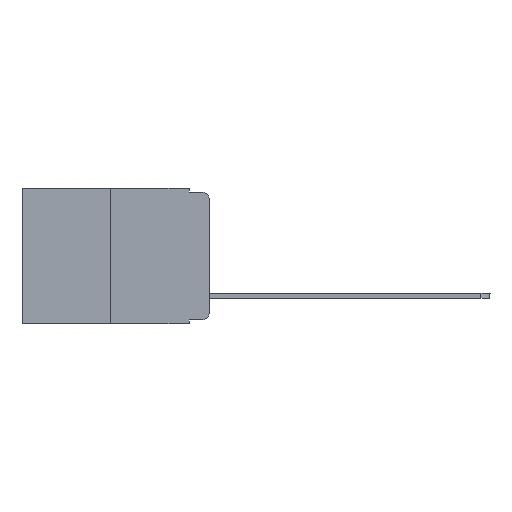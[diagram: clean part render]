
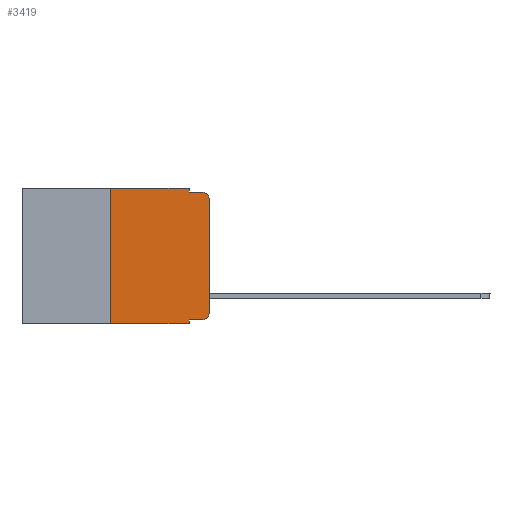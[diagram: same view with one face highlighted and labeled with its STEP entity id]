
A CAD part, left-side view. The second image highlights one B-rep face of the part: STEP entity #3419.
In plain terms, the highlighted planar face has unit normal (-1, 0, 0).
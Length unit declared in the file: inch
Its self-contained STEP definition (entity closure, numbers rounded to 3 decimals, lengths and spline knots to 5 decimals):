
#386 = DIRECTION ( 'NONE',  ( 0., -1., 0. ) ) ;
#850 = ORIENTED_EDGE ( 'NONE', *, *, #2963, .F. ) ;
#1186 = CARTESIAN_POINT ( 'NONE',  ( 0., 0.02, -0.333 ) ) ;
#1317 = VERTEX_POINT ( 'NONE', #8424 ) ;
#1328 = CARTESIAN_POINT ( 'NONE',  ( 0., 0.02, -0.313 ) ) ;
#1638 = AXIS2_PLACEMENT_3D ( 'NONE', #11266, #3625, #21027 ) ;
#1737 = DIRECTION ( 'NONE',  ( 0., 0., -1. ) ) ;
#1816 = PLANE ( 'NONE',  #14323 ) ;
#2111 = CARTESIAN_POINT ( 'NONE',  ( 0., 0.473, 0. ) ) ;
#2673 = VECTOR ( 'NONE', #6507, 39.37008 ) ;
#2772 = EDGE_CURVE ( 'NONE', #17605, #16877, #12616, .T. ) ;
#2912 = LINE ( 'NONE', #18520, #10116 ) ;
#2963 = EDGE_CURVE ( 'NONE', #8290, #1317, #24633, .T. ) ;
#3319 = CARTESIAN_POINT ( 'NONE',  ( 0., 0.25, -0.343 ) ) ;
#3368 = LINE ( 'NONE', #15647, #24435 ) ;
#3419 = ADVANCED_FACE ( 'NONE', ( #14100 ), #1816, .F. ) ;
#3489 = ORIENTED_EDGE ( 'NONE', *, *, #8523, .F. ) ;
#3625 = DIRECTION ( 'NONE',  ( -1., 0., 0. ) ) ;
#3786 = ORIENTED_EDGE ( 'NONE', *, *, #5495, .T. ) ;
#3880 = VERTEX_POINT ( 'NONE', #7819 ) ;
#4097 = VERTEX_POINT ( 'NONE', #4780 ) ;
#4254 = VECTOR ( 'NONE', #16210, 39.37008 ) ;
#4737 = CARTESIAN_POINT ( 'NONE',  ( 0., 0., -0.03 ) ) ;
#4780 = CARTESIAN_POINT ( 'NONE',  ( 0., 0.02, -0.01 ) ) ;
#4804 = ORIENTED_EDGE ( 'NONE', *, *, #19034, .T. ) ;
#5077 = EDGE_CURVE ( 'NONE', #17605, #7780, #19011, .T. ) ;
#5107 = DIRECTION ( 'NONE',  ( -1., 0., 0. ) ) ;
#5423 = CARTESIAN_POINT ( 'NONE',  ( 0., 0.473, 0. ) ) ;
#5495 = EDGE_CURVE ( 'NONE', #16734, #4097, #6612, .T. ) ;
#6049 = VERTEX_POINT ( 'NONE', #13752 ) ;
#6392 = ORIENTED_EDGE ( 'NONE', *, *, #20083, .F. ) ;
#6507 = DIRECTION ( 'NONE',  ( 0., -1., 0. ) ) ;
#6580 = AXIS2_PLACEMENT_3D ( 'NONE', #1328, #5107, #6944 ) ;
#6612 = CIRCLE ( 'NONE', #1638, 0.02 ) ;
#6631 = VECTOR ( 'NONE', #13876, 39.37008 ) ;
#6944 = DIRECTION ( 'NONE',  ( 0., 0., -1. ) ) ;
#7354 = DIRECTION ( 'NONE',  ( 1., 0., 0. ) ) ;
#7780 = VERTEX_POINT ( 'NONE', #8704 ) ;
#7819 = CARTESIAN_POINT ( 'NONE',  ( 0., 0., -0.313 ) ) ;
#8290 = VERTEX_POINT ( 'NONE', #13399 ) ;
#8424 = CARTESIAN_POINT ( 'NONE',  ( 0., 0.051, 0. ) ) ;
#8523 = EDGE_CURVE ( 'NONE', #9885, #8290, #14919, .T. ) ;
#8704 = CARTESIAN_POINT ( 'NONE',  ( 0., 0.051, -0.343 ) ) ;
#8719 = ORIENTED_EDGE ( 'NONE', *, *, #17128, .F. ) ;
#9520 = DIRECTION ( 'NONE',  ( 0., 0., -1. ) ) ;
#9591 = VECTOR ( 'NONE', #11482, 39.37008 ) ;
#9613 = VECTOR ( 'NONE', #15052, 39.37008 ) ;
#9885 = VERTEX_POINT ( 'NONE', #3319 ) ;
#10116 = VECTOR ( 'NONE', #9520, 39.37008 ) ;
#11083 = CARTESIAN_POINT ( 'NONE',  ( 0., 0.051, -0.333 ) ) ;
#11266 = CARTESIAN_POINT ( 'NONE',  ( 0., 0.02, -0.03 ) ) ;
#11288 = CIRCLE ( 'NONE', #6580, 0.02 ) ;
#11372 = LINE ( 'NONE', #16880, #9591 ) ;
#11482 = DIRECTION ( 'NONE',  ( 0., 0., 1. ) ) ;
#11768 = LINE ( 'NONE', #16019, #6631 ) ;
#12616 = LINE ( 'NONE', #13467, #9613 ) ;
#13399 = CARTESIAN_POINT ( 'NONE',  ( 0., 0.25, 0. ) ) ;
#13467 = CARTESIAN_POINT ( 'NONE',  ( 0., 0.051, -0.333 ) ) ;
#13752 = CARTESIAN_POINT ( 'NONE',  ( 0., 0.051, -0.01 ) ) ;
#13791 = CARTESIAN_POINT ( 'NONE',  ( 0., 0.051, 0. ) ) ;
#13815 = ORIENTED_EDGE ( 'NONE', *, *, #5077, .F. ) ;
#13876 = DIRECTION ( 'NONE',  ( 0., -1., 0. ) ) ;
#14100 = FACE_OUTER_BOUND ( 'NONE', #17581, .T. ) ;
#14323 = AXIS2_PLACEMENT_3D ( 'NONE', #5423, #7354, #1737 ) ;
#14362 = EDGE_CURVE ( 'NONE', #16877, #3880, #11288, .T. ) ;
#14628 = VECTOR ( 'NONE', #15766, 39.37008 ) ;
#14919 = LINE ( 'NONE', #21642, #14628 ) ;
#15052 = DIRECTION ( 'NONE',  ( 0., -1., 0. ) ) ;
#15647 = CARTESIAN_POINT ( 'NONE',  ( 0., 0.051, -0.01 ) ) ;
#15766 = DIRECTION ( 'NONE',  ( 0., 0., 1. ) ) ;
#16019 = CARTESIAN_POINT ( 'NONE',  ( 0., 0.473, -0.343 ) ) ;
#16210 = DIRECTION ( 'NONE',  ( 0., 0., -1. ) ) ;
#16734 = VERTEX_POINT ( 'NONE', #4737 ) ;
#16877 = VERTEX_POINT ( 'NONE', #1186 ) ;
#16880 = CARTESIAN_POINT ( 'NONE',  ( 0., 0., 0. ) ) ;
#17128 = EDGE_CURVE ( 'NONE', #6049, #4097, #3368, .T. ) ;
#17581 = EDGE_LOOP ( 'NONE', ( #4804, #3786, #8719, #6392, #850, #3489, #19554, #13815, #22152, #23320 ) ) ;
#17605 = VERTEX_POINT ( 'NONE', #11083 ) ;
#17926 = EDGE_CURVE ( 'NONE', #9885, #7780, #11768, .T. ) ;
#18520 = CARTESIAN_POINT ( 'NONE',  ( 0., 0.051, 0. ) ) ;
#19011 = LINE ( 'NONE', #13791, #4254 ) ;
#19034 = EDGE_CURVE ( 'NONE', #3880, #16734, #11372, .T. ) ;
#19554 = ORIENTED_EDGE ( 'NONE', *, *, #17926, .T. ) ;
#20083 = EDGE_CURVE ( 'NONE', #1317, #6049, #2912, .T. ) ;
#21027 = DIRECTION ( 'NONE',  ( 0., 0., -1. ) ) ;
#21642 = CARTESIAN_POINT ( 'NONE',  ( 0., 0.25, 0. ) ) ;
#22152 = ORIENTED_EDGE ( 'NONE', *, *, #2772, .T. ) ;
#23320 = ORIENTED_EDGE ( 'NONE', *, *, #14362, .T. ) ;
#24435 = VECTOR ( 'NONE', #386, 39.37008 ) ;
#24633 = LINE ( 'NONE', #2111, #2673 ) ;
